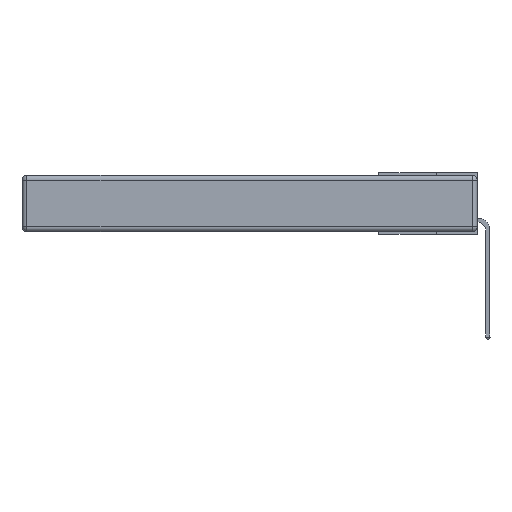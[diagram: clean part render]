
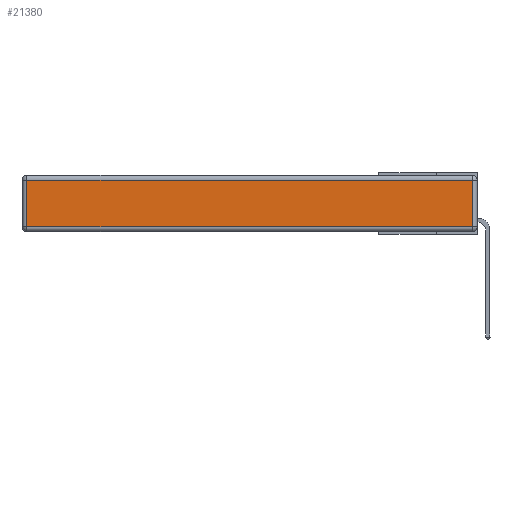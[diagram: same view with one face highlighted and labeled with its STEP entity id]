
A CAD part, left-side view. The second image highlights one B-rep face of the part: STEP entity #21380.
In plain terms, the highlighted planar face has unit normal (-1, 0, 0).
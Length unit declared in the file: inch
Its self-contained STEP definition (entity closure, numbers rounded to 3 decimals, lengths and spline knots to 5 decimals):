
#321 = CARTESIAN_POINT ( 'NONE',  ( 0., 0., -0.313 ) ) ;
#1954 = EDGE_CURVE ( 'NONE', #11636, #22430, #23222, .T. ) ;
#2691 = EDGE_LOOP ( 'NONE', ( #8367, #19872, #28005, #26084 ) ) ;
#3789 = DIRECTION ( 'NONE',  ( 0., 0., 1. ) ) ;
#5065 = VERTEX_POINT ( 'NONE', #5439 ) ;
#5326 = LINE ( 'NONE', #29354, #28331 ) ;
#5439 = CARTESIAN_POINT ( 'NONE',  ( 0., 0.03, -0.03 ) ) ;
#5954 = PLANE ( 'NONE',  #10321 ) ;
#6067 = DIRECTION ( 'NONE',  ( -1., 0., 0. ) ) ;
#7389 = DIRECTION ( 'NONE',  ( 0., 0., 1. ) ) ;
#8367 = ORIENTED_EDGE ( 'NONE', *, *, #1954, .T. ) ;
#10321 = AXIS2_PLACEMENT_3D ( 'NONE', #13899, #6067, #3789 ) ;
#11080 = DIRECTION ( 'NONE',  ( 0., 1., 0. ) ) ;
#11636 = VERTEX_POINT ( 'NONE', #17932 ) ;
#13407 = DIRECTION ( 'NONE',  ( 0., 0., -1. ) ) ;
#13899 = CARTESIAN_POINT ( 'NONE',  ( 0., 0., -0.343 ) ) ;
#14819 = EDGE_CURVE ( 'NONE', #24979, #11636, #5326, .T. ) ;
#16209 = VECTOR ( 'NONE', #23527, 39.37008 ) ;
#16505 = EDGE_CURVE ( 'NONE', #5065, #24979, #32787, .T. ) ;
#17932 = CARTESIAN_POINT ( 'NONE',  ( 0., 2.72, -0.313 ) ) ;
#17955 = VECTOR ( 'NONE', #11080, 39.37008 ) ;
#19106 = CARTESIAN_POINT ( 'NONE',  ( 0., 2.72, -0.03 ) ) ;
#19584 = CARTESIAN_POINT ( 'NONE',  ( 0., 0.03, -0.313 ) ) ;
#19872 = ORIENTED_EDGE ( 'NONE', *, *, #25796, .T. ) ;
#20327 = VECTOR ( 'NONE', #7389, 39.37008 ) ;
#20528 = CARTESIAN_POINT ( 'NONE',  ( 0., 0.03, -0.343 ) ) ;
#21380 = ADVANCED_FACE ( 'NONE', ( #28393 ), #5954, .T. ) ;
#22430 = VERTEX_POINT ( 'NONE', #19584 ) ;
#23222 = LINE ( 'NONE', #321, #16209 ) ;
#23527 = DIRECTION ( 'NONE',  ( 0., -1., 0. ) ) ;
#24979 = VERTEX_POINT ( 'NONE', #19106 ) ;
#25796 = EDGE_CURVE ( 'NONE', #22430, #5065, #26049, .T. ) ;
#26049 = LINE ( 'NONE', #20528, #20327 ) ;
#26084 = ORIENTED_EDGE ( 'NONE', *, *, #14819, .T. ) ;
#26609 = CARTESIAN_POINT ( 'NONE',  ( 0., 2.75, -0.03 ) ) ;
#28005 = ORIENTED_EDGE ( 'NONE', *, *, #16505, .T. ) ;
#28331 = VECTOR ( 'NONE', #13407, 39.37008 ) ;
#28393 = FACE_OUTER_BOUND ( 'NONE', #2691, .T. ) ;
#29354 = CARTESIAN_POINT ( 'NONE',  ( 0., 2.72, -0.343 ) ) ;
#32787 = LINE ( 'NONE', #26609, #17955 ) ;
